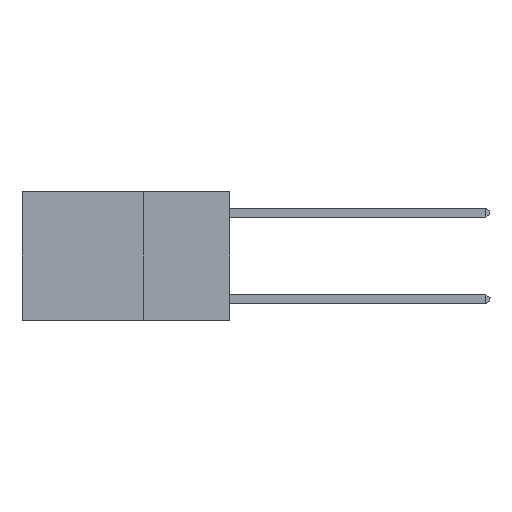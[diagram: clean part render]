
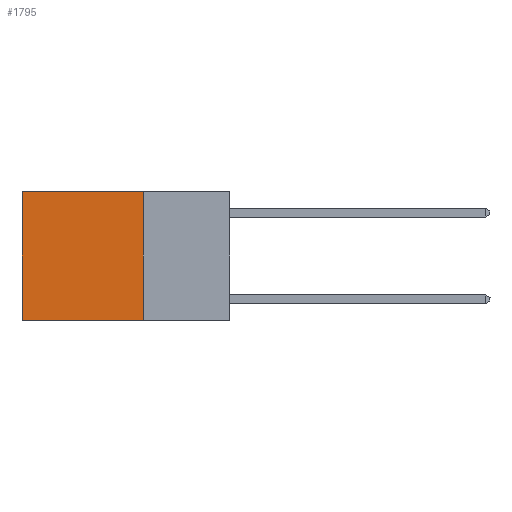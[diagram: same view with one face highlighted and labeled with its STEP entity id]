
A CAD part, left-side view. The second image highlights one B-rep face of the part: STEP entity #1795.
In plain terms, the highlighted planar face has unit normal (-1, 0, 0).
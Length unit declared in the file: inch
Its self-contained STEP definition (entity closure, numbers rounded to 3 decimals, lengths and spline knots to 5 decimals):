
#206 = DIRECTION ( 'NONE',  ( 0., 0., -1. ) ) ;
#1795 = ADVANCED_FACE ( 'NONE', ( #15845 ), #4377, .F. ) ;
#2020 = EDGE_LOOP ( 'NONE', ( #19940, #4396, #13899, #7187 ) ) ;
#3728 = LINE ( 'NONE', #20869, #20524 ) ;
#3738 = VERTEX_POINT ( 'NONE', #20362 ) ;
#3857 = CARTESIAN_POINT ( 'NONE',  ( 0.2625, 0.25, -0.37 ) ) ;
#4266 = VECTOR ( 'NONE', #13209, 39.37008 ) ;
#4377 = PLANE ( 'NONE',  #7647 ) ;
#4396 = ORIENTED_EDGE ( 'NONE', *, *, #23966, .F. ) ;
#4851 = CARTESIAN_POINT ( 'NONE',  ( 0.2625, 0.25, 0. ) ) ;
#5690 = VERTEX_POINT ( 'NONE', #9232 ) ;
#5842 = LINE ( 'NONE', #3857, #17515 ) ;
#7187 = ORIENTED_EDGE ( 'NONE', *, *, #18267, .T. ) ;
#7647 = AXIS2_PLACEMENT_3D ( 'NONE', #4851, #23374, #11909 ) ;
#7917 = VERTEX_POINT ( 'NONE', #16214 ) ;
#8140 = EDGE_CURVE ( 'NONE', #17759, #3738, #3728, .T. ) ;
#9232 = CARTESIAN_POINT ( 'NONE',  ( 0.2625, 0.6, -0.37 ) ) ;
#10270 = CARTESIAN_POINT ( 'NONE',  ( 0.2625, 0.25, 0. ) ) ;
#11690 = LINE ( 'NONE', #13043, #23443 ) ;
#11909 = DIRECTION ( 'NONE',  ( 0., 0., -1. ) ) ;
#12110 = EDGE_CURVE ( 'NONE', #7917, #5690, #11690, .T. ) ;
#13043 = CARTESIAN_POINT ( 'NONE',  ( 0.2625, 0.6, 0. ) ) ;
#13209 = DIRECTION ( 'NONE',  ( 0., 1., 0. ) ) ;
#13331 = LINE ( 'NONE', #23073, #4266 ) ;
#13899 = ORIENTED_EDGE ( 'NONE', *, *, #8140, .F. ) ;
#15845 = FACE_OUTER_BOUND ( 'NONE', #2020, .T. ) ;
#16214 = CARTESIAN_POINT ( 'NONE',  ( 0.2625, 0.6, 0. ) ) ;
#16566 = DIRECTION ( 'NONE',  ( 0., 1., 0. ) ) ;
#17515 = VECTOR ( 'NONE', #16566, 39.37008 ) ;
#17759 = VERTEX_POINT ( 'NONE', #10270 ) ;
#18267 = EDGE_CURVE ( 'NONE', #17759, #7917, #13331, .T. ) ;
#19940 = ORIENTED_EDGE ( 'NONE', *, *, #12110, .T. ) ;
#20362 = CARTESIAN_POINT ( 'NONE',  ( 0.2625, 0.25, -0.37 ) ) ;
#20524 = VECTOR ( 'NONE', #24220, 39.37008 ) ;
#20869 = CARTESIAN_POINT ( 'NONE',  ( 0.2625, 0.25, 0. ) ) ;
#23073 = CARTESIAN_POINT ( 'NONE',  ( 0.2625, 0.25, 0. ) ) ;
#23374 = DIRECTION ( 'NONE',  ( 1., 0., 0. ) ) ;
#23443 = VECTOR ( 'NONE', #206, 39.37008 ) ;
#23966 = EDGE_CURVE ( 'NONE', #3738, #5690, #5842, .T. ) ;
#24220 = DIRECTION ( 'NONE',  ( 0., 0., -1. ) ) ;
